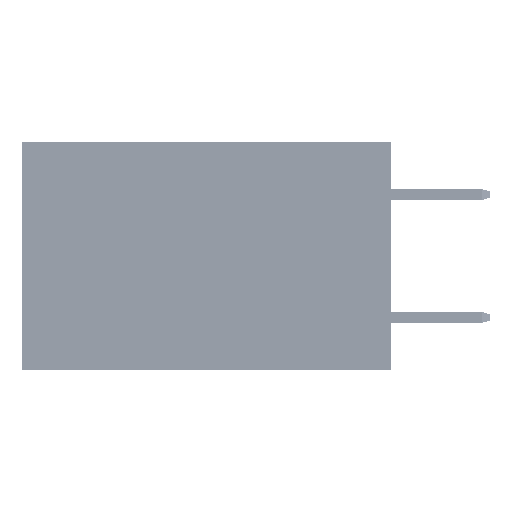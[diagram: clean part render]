
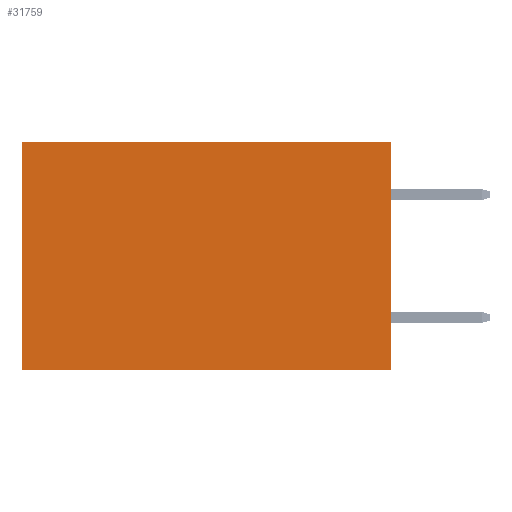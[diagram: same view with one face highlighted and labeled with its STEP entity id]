
A CAD part, left-side view. The second image highlights one B-rep face of the part: STEP entity #31759.
In plain terms, the highlighted planar face has unit normal (-1, 0, 0).
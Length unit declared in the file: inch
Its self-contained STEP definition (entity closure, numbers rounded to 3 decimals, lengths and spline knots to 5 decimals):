
#579 = AXIS2_PLACEMENT_3D ( 'NONE', #25771, #5838, #25599 ) ;
#851 = VERTEX_POINT ( 'NONE', #14868 ) ;
#1628 = ORIENTED_EDGE ( 'NONE', *, *, #4413, .F. ) ;
#3850 = VECTOR ( 'NONE', #45686, 39.37008 ) ;
#3957 = DIRECTION ( 'NONE',  ( 0., 0., -1. ) ) ;
#4102 = CARTESIAN_POINT ( 'NONE',  ( 0.2875, 0., -0.37 ) ) ;
#4413 = EDGE_CURVE ( 'NONE', #11035, #48199, #31729, .T. ) ;
#5838 = DIRECTION ( 'NONE',  ( 1., 0., 0. ) ) ;
#10041 = DIRECTION ( 'NONE',  ( 0., 1., 0. ) ) ;
#10727 = PLANE ( 'NONE',  #579 ) ;
#10826 = LINE ( 'NONE', #19194, #3850 ) ;
#11035 = VERTEX_POINT ( 'NONE', #27480 ) ;
#13628 = VECTOR ( 'NONE', #38237, 39.37008 ) ;
#13666 = CARTESIAN_POINT ( 'NONE',  ( 0.2875, 0., 0. ) ) ;
#14868 = CARTESIAN_POINT ( 'NONE',  ( 0.2875, 0.6, 0. ) ) ;
#16009 = CARTESIAN_POINT ( 'NONE',  ( 0.2875, 0., 0. ) ) ;
#17590 = VECTOR ( 'NONE', #3957, 39.37008 ) ;
#18433 = CARTESIAN_POINT ( 'NONE',  ( 0.2875, 0., 0. ) ) ;
#19194 = CARTESIAN_POINT ( 'NONE',  ( 0.2875, 0.6, 0. ) ) ;
#19828 = CARTESIAN_POINT ( 'NONE',  ( 0.2875, 0.6, -0.37 ) ) ;
#19838 = VECTOR ( 'NONE', #10041, 39.37008 ) ;
#21402 = ORIENTED_EDGE ( 'NONE', *, *, #29345, .F. ) ;
#22698 = VERTEX_POINT ( 'NONE', #16009 ) ;
#25599 = DIRECTION ( 'NONE',  ( 0., 0., -1. ) ) ;
#25771 = CARTESIAN_POINT ( 'NONE',  ( 0.2875, 0., 0. ) ) ;
#26649 = FACE_OUTER_BOUND ( 'NONE', #31825, .T. ) ;
#27480 = CARTESIAN_POINT ( 'NONE',  ( 0.2875, 0., -0.37 ) ) ;
#29345 = EDGE_CURVE ( 'NONE', #22698, #11035, #42727, .T. ) ;
#31250 = ORIENTED_EDGE ( 'NONE', *, *, #35546, .T. ) ;
#31729 = LINE ( 'NONE', #4102, #13628 ) ;
#31759 = ADVANCED_FACE ( 'NONE', ( #26649 ), #10727, .F. ) ;
#31825 = EDGE_LOOP ( 'NONE', ( #43638, #1628, #21402, #31250 ) ) ;
#32187 = EDGE_CURVE ( 'NONE', #851, #48199, #10826, .T. ) ;
#35546 = EDGE_CURVE ( 'NONE', #22698, #851, #38571, .T. ) ;
#38237 = DIRECTION ( 'NONE',  ( 0., 1., 0. ) ) ;
#38571 = LINE ( 'NONE', #13666, #19838 ) ;
#42727 = LINE ( 'NONE', #18433, #17590 ) ;
#43638 = ORIENTED_EDGE ( 'NONE', *, *, #32187, .T. ) ;
#45686 = DIRECTION ( 'NONE',  ( 0., 0., -1. ) ) ;
#48199 = VERTEX_POINT ( 'NONE', #19828 ) ;
